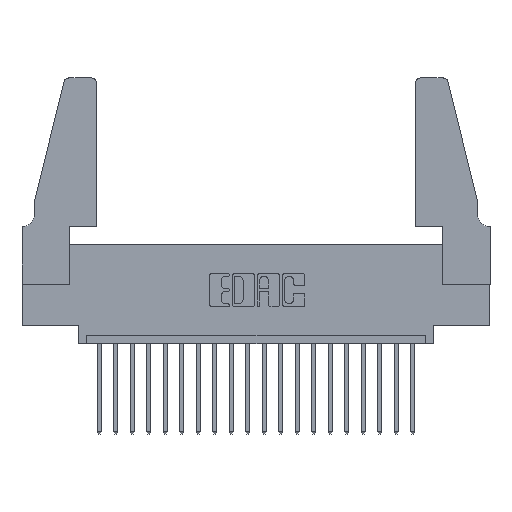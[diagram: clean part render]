
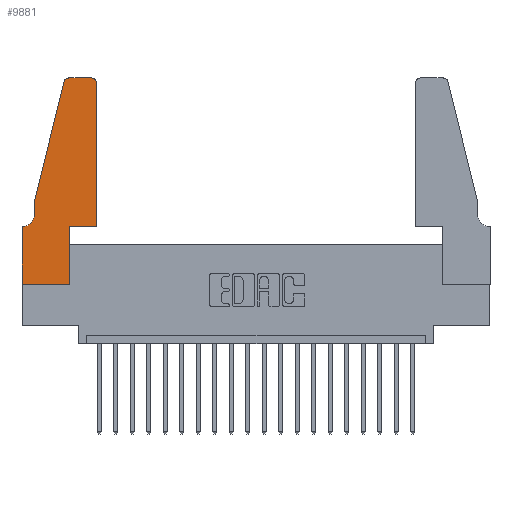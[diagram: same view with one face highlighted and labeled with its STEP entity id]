
A CAD part, top view. The second image highlights one B-rep face of the part: STEP entity #9881.
In plain terms, the highlighted planar face has unit normal (0, 0, 1).
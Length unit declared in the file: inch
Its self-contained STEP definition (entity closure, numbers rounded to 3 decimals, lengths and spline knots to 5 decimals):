
#46 = VECTOR ( 'NONE', #8863, 39.37008 ) ;
#141 = CARTESIAN_POINT ( 'NONE',  ( 0.4505, 0.35, 0.37 ) ) ;
#391 = LINE ( 'NONE', #12435, #16603 ) ;
#413 = CIRCLE ( 'NONE', #10745, 0.03 ) ;
#761 = EDGE_LOOP ( 'NONE', ( #11476, #1032, #8687, #2623, #13513, #9319, #11826, #10290, #20178, #5177, #4919, #782 ) ) ;
#782 = ORIENTED_EDGE ( 'NONE', *, *, #10541, .T. ) ;
#874 = AXIS2_PLACEMENT_3D ( 'NONE', #4307, #7116, #10503 ) ;
#1032 = ORIENTED_EDGE ( 'NONE', *, *, #6466, .T. ) ;
#1059 = VERTEX_POINT ( 'NONE', #2994 ) ;
#1248 = CARTESIAN_POINT ( 'NONE',  ( 0.0755, 0.5, 0.37 ) ) ;
#1655 = VECTOR ( 'NONE', #5034, 39.37008 ) ;
#1712 = DIRECTION ( 'NONE',  ( -1., 0., 0. ) ) ;
#1727 = AXIS2_PLACEMENT_3D ( 'NONE', #7435, #7780, #3124 ) ;
#1800 = VECTOR ( 'NONE', #14241, 39.37008 ) ;
#2173 = CARTESIAN_POINT ( 'NONE',  ( 0.25487, 1.22718, 0.37 ) ) ;
#2174 = VERTEX_POINT ( 'NONE', #16462 ) ;
#2516 = CARTESIAN_POINT ( 'NONE',  ( 0.4205, 1.22, 0.37 ) ) ;
#2571 = CARTESIAN_POINT ( 'NONE',  ( 0.0055, 0.35, 0.37 ) ) ;
#2623 = ORIENTED_EDGE ( 'NONE', *, *, #7715, .T. ) ;
#2994 = CARTESIAN_POINT ( 'NONE',  ( 0.0755, 0.42, 0.37 ) ) ;
#3124 = DIRECTION ( 'NONE',  ( -1., 0., 0. ) ) ;
#3402 = EDGE_CURVE ( 'NONE', #4941, #10710, #13581, .T. ) ;
#3617 = LINE ( 'NONE', #7057, #12167 ) ;
#3698 = LINE ( 'NONE', #13499, #13700 ) ;
#3789 = AXIS2_PLACEMENT_3D ( 'NONE', #7901, #7773, #6337 ) ;
#4307 = CARTESIAN_POINT ( 'NONE',  ( 0., 0.35, 0.37 ) ) ;
#4393 = EDGE_CURVE ( 'NONE', #9921, #4941, #5487, .T. ) ;
#4522 = VERTEX_POINT ( 'NONE', #2571 ) ;
#4919 = ORIENTED_EDGE ( 'NONE', *, *, #3402, .T. ) ;
#4941 = VERTEX_POINT ( 'NONE', #16984 ) ;
#5034 = DIRECTION ( 'NONE',  ( 1., 0., 0. ) ) ;
#5177 = ORIENTED_EDGE ( 'NONE', *, *, #4393, .T. ) ;
#5418 = CIRCLE ( 'NONE', #3789, 0.03 ) ;
#5487 = LINE ( 'NONE', #20274, #19443 ) ;
#5672 = DIRECTION ( 'NONE',  ( 0., 0., 1. ) ) ;
#5875 = LINE ( 'NONE', #9592, #1655 ) ;
#6337 = DIRECTION ( 'NONE',  ( 1., 0., 0. ) ) ;
#6466 = EDGE_CURVE ( 'NONE', #20220, #18107, #5418, .T. ) ;
#6552 = VECTOR ( 'NONE', #12216, 39.37008 ) ;
#7057 = CARTESIAN_POINT ( 'NONE',  ( 0.2865, 0.35, 0.37 ) ) ;
#7116 = DIRECTION ( 'NONE',  ( 0., 0., 1. ) ) ;
#7172 = EDGE_CURVE ( 'NONE', #2174, #12179, #5875, .T. ) ;
#7435 = CARTESIAN_POINT ( 'NONE',  ( 0.0055, 0.42, 0.37 ) ) ;
#7715 = EDGE_CURVE ( 'NONE', #18152, #1059, #11904, .T. ) ;
#7773 = DIRECTION ( 'NONE',  ( 0., 0., 1. ) ) ;
#7780 = DIRECTION ( 'NONE',  ( 0., 0., -1. ) ) ;
#7901 = CARTESIAN_POINT ( 'NONE',  ( 0.284, 1.22, 0.37 ) ) ;
#7953 = CARTESIAN_POINT ( 'NONE',  ( 0.0755, 0.5, 0.37 ) ) ;
#8329 = CARTESIAN_POINT ( 'NONE',  ( 0.4205, 1.25, 0.37 ) ) ;
#8630 = DIRECTION ( 'NONE',  ( 0., 1., 0. ) ) ;
#8687 = ORIENTED_EDGE ( 'NONE', *, *, #13363, .T. ) ;
#8863 = DIRECTION ( 'NONE',  ( 0., -1., 0. ) ) ;
#9319 = ORIENTED_EDGE ( 'NONE', *, *, #19945, .T. ) ;
#9592 = CARTESIAN_POINT ( 'NONE',  ( 0., 0., 0.37 ) ) ;
#9881 = ADVANCED_FACE ( 'NONE', ( #15915 ), #16641, .T. ) ;
#9921 = VERTEX_POINT ( 'NONE', #10438 ) ;
#10028 = DIRECTION ( 'NONE',  ( -1., 0., 0. ) ) ;
#10290 = ORIENTED_EDGE ( 'NONE', *, *, #7172, .T. ) ;
#10438 = CARTESIAN_POINT ( 'NONE',  ( 0.2865, 0.35, 0.37 ) ) ;
#10503 = DIRECTION ( 'NONE',  ( 1., 0., 0. ) ) ;
#10541 = EDGE_CURVE ( 'NONE', #10710, #17778, #413, .T. ) ;
#10710 = VERTEX_POINT ( 'NONE', #11880 ) ;
#10745 = AXIS2_PLACEMENT_3D ( 'NONE', #2516, #5672, #15119 ) ;
#10755 = EDGE_CURVE ( 'NONE', #12179, #9921, #3617, .T. ) ;
#10896 = EDGE_CURVE ( 'NONE', #17778, #20220, #391, .T. ) ;
#11109 = DIRECTION ( 'NONE',  ( 0., 1., 0. ) ) ;
#11237 = CARTESIAN_POINT ( 'NONE',  ( 0.284, 1.25, 0.37 ) ) ;
#11476 = ORIENTED_EDGE ( 'NONE', *, *, #10896, .T. ) ;
#11657 = EDGE_CURVE ( 'NONE', #1059, #4522, #18265, .T. ) ;
#11727 = VERTEX_POINT ( 'NONE', #17223 ) ;
#11826 = ORIENTED_EDGE ( 'NONE', *, *, #18517, .T. ) ;
#11880 = CARTESIAN_POINT ( 'NONE',  ( 0.4505, 1.22, 0.37 ) ) ;
#11904 = LINE ( 'NONE', #1248, #6552 ) ;
#12167 = VECTOR ( 'NONE', #8630, 39.37008 ) ;
#12179 = VERTEX_POINT ( 'NONE', #17873 ) ;
#12216 = DIRECTION ( 'NONE',  ( 0., -1., 0. ) ) ;
#12435 = CARTESIAN_POINT ( 'NONE',  ( 0.2605, 1.25, 0.37 ) ) ;
#13363 = EDGE_CURVE ( 'NONE', #18107, #18152, #18949, .T. ) ;
#13499 = CARTESIAN_POINT ( 'NONE',  ( 0.0755, 0.35, 0.37 ) ) ;
#13513 = ORIENTED_EDGE ( 'NONE', *, *, #11657, .T. ) ;
#13581 = LINE ( 'NONE', #141, #16074 ) ;
#13700 = VECTOR ( 'NONE', #10028, 39.37008 ) ;
#14241 = DIRECTION ( 'NONE',  ( -0.239, -0.971, 0. ) ) ;
#15119 = DIRECTION ( 'NONE',  ( 1., 0., 0. ) ) ;
#15751 = DIRECTION ( 'NONE',  ( 1., 0., 0. ) ) ;
#15915 = FACE_OUTER_BOUND ( 'NONE', #761, .T. ) ;
#16074 = VECTOR ( 'NONE', #11109, 39.37008 ) ;
#16462 = CARTESIAN_POINT ( 'NONE',  ( 0., 0., 0.37 ) ) ;
#16603 = VECTOR ( 'NONE', #1712, 39.37008 ) ;
#16641 = PLANE ( 'NONE',  #874 ) ;
#16984 = CARTESIAN_POINT ( 'NONE',  ( 0.4505, 0.35, 0.37 ) ) ;
#17223 = CARTESIAN_POINT ( 'NONE',  ( 0., 0.35, 0.37 ) ) ;
#17653 = CARTESIAN_POINT ( 'NONE',  ( 0., 0., 0.37 ) ) ;
#17778 = VERTEX_POINT ( 'NONE', #8329 ) ;
#17873 = CARTESIAN_POINT ( 'NONE',  ( 0.2865, 0., 0.37 ) ) ;
#17986 = CARTESIAN_POINT ( 'NONE',  ( 0.0755, 0.5, 0.37 ) ) ;
#18107 = VERTEX_POINT ( 'NONE', #2173 ) ;
#18152 = VERTEX_POINT ( 'NONE', #17986 ) ;
#18265 = CIRCLE ( 'NONE', #1727, 0.07 ) ;
#18464 = LINE ( 'NONE', #17653, #46 ) ;
#18517 = EDGE_CURVE ( 'NONE', #11727, #2174, #18464, .T. ) ;
#18949 = LINE ( 'NONE', #7953, #1800 ) ;
#19443 = VECTOR ( 'NONE', #15751, 39.37008 ) ;
#19945 = EDGE_CURVE ( 'NONE', #4522, #11727, #3698, .T. ) ;
#20178 = ORIENTED_EDGE ( 'NONE', *, *, #10755, .T. ) ;
#20220 = VERTEX_POINT ( 'NONE', #11237 ) ;
#20274 = CARTESIAN_POINT ( 'NONE',  ( 0.4505, 0.35, 0.37 ) ) ;
